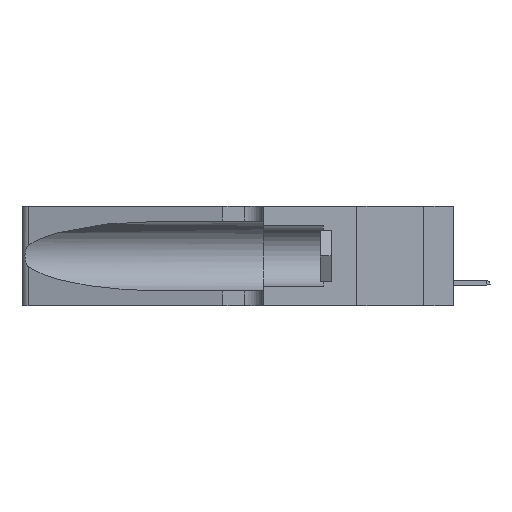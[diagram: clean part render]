
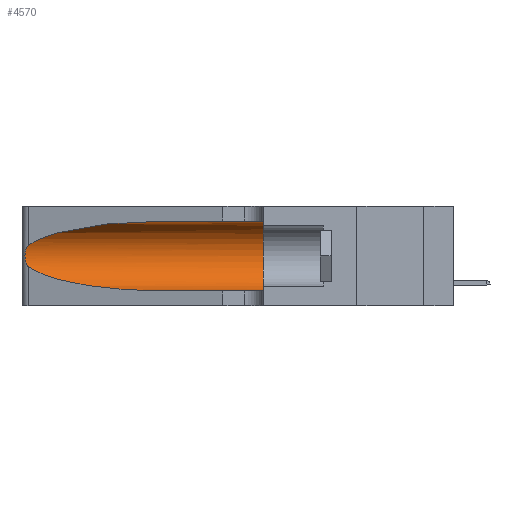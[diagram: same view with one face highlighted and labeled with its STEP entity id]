
A CAD part, left-side view. The second image highlights one B-rep face of the part: STEP entity #4570.
In plain terms, the highlighted cylindrical face has radius 3.308 mm (diameter 6.617 mm), a partial arc.
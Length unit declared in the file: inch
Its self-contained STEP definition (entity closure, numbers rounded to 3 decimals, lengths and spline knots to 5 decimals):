
#245 = CARTESIAN_POINT ( 'NONE',  ( 0.18966, 0.96281, 0.31525 ) ) ;
#310 = CARTESIAN_POINT ( 'NONE',  ( 0.1305, 0.72297, 0.05475 ) ) ;
#1001 = LINE ( 'NONE', #11052, #7367 ) ;
#1384 = LINE ( 'NONE', #14060, #7522 ) ;
#1678 = VERTEX_POINT ( 'NONE', #14768 ) ;
#1767 = DIRECTION ( 'NONE',  ( 0., 0., -1. ) ) ;
#2031 = FACE_OUTER_BOUND ( 'NONE', #14186, .T. ) ;
#3144 = AXIS2_PLACEMENT_3D ( 'NONE', #3240, #10675, #1767 ) ;
#3240 = CARTESIAN_POINT ( 'NONE',  ( 0.1305, 1.61858, 0.185 ) ) ;
#3788 = CARTESIAN_POINT ( 'NONE',  ( 0.25487, 1.22718, 0.22369 ) ) ;
#3961 = CARTESIAN_POINT ( 'NONE',  ( 0.25856, 1.23593, 0.16098 ) ) ;
#4228 = DIRECTION ( 'NONE',  ( 0., 0., 1. ) ) ;
#4570 = ADVANCED_FACE ( 'NONE', ( #2031 ), #7749, .F. ) ;
#4572 = CARTESIAN_POINT ( 'NONE',  ( 0.18966, 0.96281, 0.05475 ) ) ;
#4682 = EDGE_CURVE ( 'NONE', #14109, #13870, #1001, .T. ) ;
#4864 = CARTESIAN_POINT ( 'NONE',  ( 0.25487, 1.22718, 0.14631 ) ) ;
#5379 = CARTESIAN_POINT ( 'NONE',  ( 0.25555, 1.22994, 0.2215 ) ) ;
#5395 = DIRECTION ( 'NONE',  ( 0., 1., 0. ) ) ;
#5465 = CARTESIAN_POINT ( 'NONE',  ( 0.25487, 1.22718, 0.14631 ) ) ;
#5528 = CIRCLE ( 'NONE', #10037, 0.13025 ) ;
#5551 = ORIENTED_EDGE ( 'NONE', *, *, #4682, .F. ) ;
#5917 = ORIENTED_EDGE ( 'NONE', *, *, #9791, .F. ) ;
#5967 = CARTESIAN_POINT ( 'NONE',  ( 0.2373, 1.15595, 0.28018 ) ) ;
#6093 = CARTESIAN_POINT ( 'NONE',  ( 0.1305, 0.72297, 0.05475 ) ) ;
#6297 = EDGE_CURVE ( 'NONE', #15476, #1678, #1384, .T. ) ;
#6608 = CARTESIAN_POINT ( 'NONE',  ( 0.1305, 0.35, 0.31525 ) ) ;
#6686 = CARTESIAN_POINT ( 'NONE',  ( 0.25639, 1.23184, 0.21858 ) ) ;
#6799 =( BOUNDED_CURVE ( )  B_SPLINE_CURVE ( 3, ( #17757, #245, #5967, #14856 ),
 .UNSPECIFIED., .F., .F. ) 
 B_SPLINE_CURVE_WITH_KNOTS ( ( 4, 4 ),
 ( 1.5708, 2.84003 ),
 .UNSPECIFIED. ) 
 CURVE ( )  GEOMETRIC_REPRESENTATION_ITEM ( )  RATIONAL_B_SPLINE_CURVE ( ( 1., 0.87, 0.87, 1. ) ) 
 REPRESENTATION_ITEM ( '' )  );
#6815 = DIRECTION ( 'NONE',  ( 0., -1., 0. ) ) ;
#7367 = VECTOR ( 'NONE', #6815, 39.37008 ) ;
#7376 = CARTESIAN_POINT ( 'NONE',  ( 0.25487, 1.22718, 0.22369 ) ) ;
#7522 = VECTOR ( 'NONE', #8498, 39.37008 ) ;
#7555 = EDGE_CURVE ( 'NONE', #10150, #15476, #16484, .T. ) ;
#7749 = CYLINDRICAL_SURFACE ( 'NONE', #3144, 0.13025 ) ;
#8233 = ORIENTED_EDGE ( 'NONE', *, *, #14687, .T. ) ;
#8498 = DIRECTION ( 'NONE',  ( 0., -1., 0. ) ) ;
#9082 = VERTEX_POINT ( 'NONE', #7376 ) ;
#9203 = ORIENTED_EDGE ( 'NONE', *, *, #11335, .T. ) ;
#9697 = CARTESIAN_POINT ( 'NONE',  ( 0.26075, 1.23896, 0.19203 ) ) ;
#9791 = EDGE_CURVE ( 'NONE', #13870, #1678, #5528, .T. ) ;
#10037 = AXIS2_PLACEMENT_3D ( 'NONE', #13942, #5395, #4228 ) ;
#10150 = VERTEX_POINT ( 'NONE', #4864 ) ;
#10675 = DIRECTION ( 'NONE',  ( 0., -1., 0. ) ) ;
#11052 = CARTESIAN_POINT ( 'NONE',  ( 0.1305, 1.61858, 0.31525 ) ) ;
#11335 = EDGE_CURVE ( 'NONE', #9082, #10150, #17254, .T. ) ;
#11634 = CARTESIAN_POINT ( 'NONE',  ( 0.2373, 1.15595, 0.08982 ) ) ;
#12235 = CARTESIAN_POINT ( 'NONE',  ( 0.25789, 1.23486, 0.15765 ) ) ;
#12330 = CARTESIAN_POINT ( 'NONE',  ( 0.26018, 1.23835, 0.19895 ) ) ;
#12427 = CARTESIAN_POINT ( 'NONE',  ( 0.25854, 1.2359, 0.20912 ) ) ;
#12520 = CARTESIAN_POINT ( 'NONE',  ( 0.26017, 1.23833, 0.17102 ) ) ;
#13870 = VERTEX_POINT ( 'NONE', #6608 ) ;
#13942 = CARTESIAN_POINT ( 'NONE',  ( 0.1305, 0.35, 0.185 ) ) ;
#14023 = CARTESIAN_POINT ( 'NONE',  ( 0.25555, 1.22993, 0.14849 ) ) ;
#14060 = CARTESIAN_POINT ( 'NONE',  ( 0.1305, 1.61858, 0.05475 ) ) ;
#14109 = VERTEX_POINT ( 'NONE', #15698 ) ;
#14186 = EDGE_LOOP ( 'NONE', ( #8233, #9203, #14369, #15361, #5917, #5551 ) ) ;
#14369 = ORIENTED_EDGE ( 'NONE', *, *, #7555, .T. ) ;
#14621 = CARTESIAN_POINT ( 'NONE',  ( 0.25487, 1.22718, 0.14631 ) ) ;
#14687 = EDGE_CURVE ( 'NONE', #14109, #9082, #6799, .T. ) ;
#14768 = CARTESIAN_POINT ( 'NONE',  ( 0.1305, 0.35, 0.05475 ) ) ;
#14856 = CARTESIAN_POINT ( 'NONE',  ( 0.25487, 1.22718, 0.22369 ) ) ;
#15361 = ORIENTED_EDGE ( 'NONE', *, *, #6297, .T. ) ;
#15424 = CARTESIAN_POINT ( 'NONE',  ( 0.25639, 1.23186, 0.15144 ) ) ;
#15476 = VERTEX_POINT ( 'NONE', #310 ) ;
#15698 = CARTESIAN_POINT ( 'NONE',  ( 0.1305, 0.72297, 0.31525 ) ) ;
#16484 =( BOUNDED_CURVE ( )  B_SPLINE_CURVE ( 3, ( #14621, #11634, #4572, #6093 ),
 .UNSPECIFIED., .F., .F. ) 
 B_SPLINE_CURVE_WITH_KNOTS ( ( 4, 4 ),
 ( 3.44316, 4.71239 ),
 .UNSPECIFIED. ) 
 CURVE ( )  GEOMETRIC_REPRESENTATION_ITEM ( )  RATIONAL_B_SPLINE_CURVE ( ( 1., 0.87, 0.87, 1. ) ) 
 REPRESENTATION_ITEM ( '' )  );
#16828 = CARTESIAN_POINT ( 'NONE',  ( 0.25787, 1.23484, 0.2124 ) ) ;
#17254 = B_SPLINE_CURVE_WITH_KNOTS ( 'NONE', 3,
 ( #3788, #5379, #6686, #16828, #12427, #12330, #9697, #18138, #12520, #3961, #12235, #15424, #14023, #5465 ),
 .UNSPECIFIED., .F., .F.,
 ( 4, 2, 2, 2, 2, 2, 4 ),
 ( 0., 0.00027, 0.00053, 0.00107, 0.0016, 0.00187, 0.00214 ),
 .UNSPECIFIED. ) ;
#17757 = CARTESIAN_POINT ( 'NONE',  ( 0.1305, 0.72297, 0.31525 ) ) ;
#18138 = CARTESIAN_POINT ( 'NONE',  ( 0.26075, 1.23896, 0.178 ) ) ;
